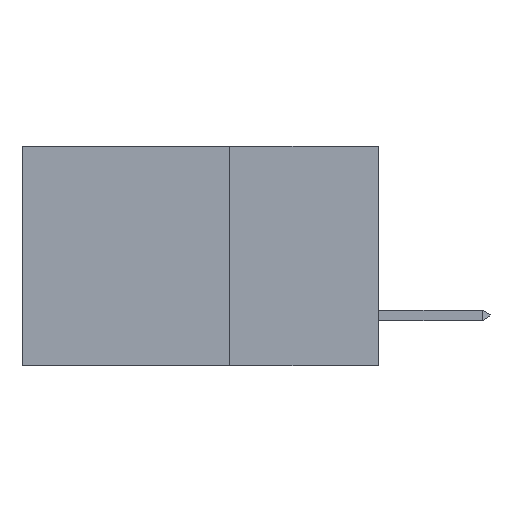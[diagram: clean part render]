
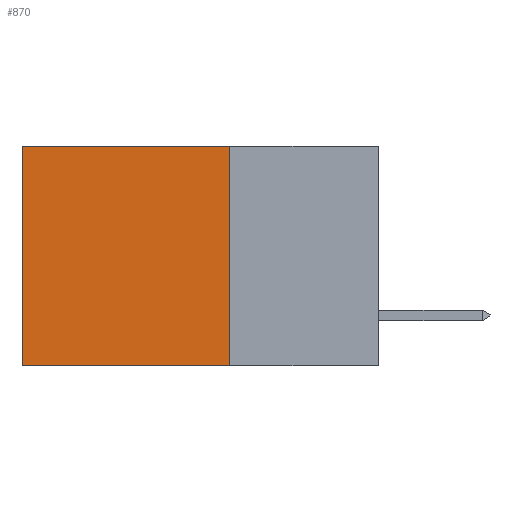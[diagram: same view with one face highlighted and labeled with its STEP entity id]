
A CAD part, left-side view. The second image highlights one B-rep face of the part: STEP entity #870.
In plain terms, the highlighted planar face has unit normal (-1, 0, 0).
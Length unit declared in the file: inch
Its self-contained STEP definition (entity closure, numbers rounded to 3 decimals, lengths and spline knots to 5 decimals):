
#489 = CARTESIAN_POINT ( 'NONE',  ( 0.2615, 0.25, -0.37 ) ) ;
#870 = ADVANCED_FACE ( 'NONE', ( #1251 ), #12846, .F. ) ;
#1251 = FACE_OUTER_BOUND ( 'NONE', #7239, .T. ) ;
#1718 = DIRECTION ( 'NONE',  ( 0., 0., -1. ) ) ;
#2157 = VERTEX_POINT ( 'NONE', #23594 ) ;
#2857 = DIRECTION ( 'NONE',  ( 0., 1., 0. ) ) ;
#4515 = VECTOR ( 'NONE', #1718, 39.37008 ) ;
#4715 = EDGE_CURVE ( 'NONE', #17413, #2157, #18904, .T. ) ;
#4854 = ORIENTED_EDGE ( 'NONE', *, *, #4715, .T. ) ;
#5540 = ORIENTED_EDGE ( 'NONE', *, *, #9986, .F. ) ;
#5983 = DIRECTION ( 'NONE',  ( 0., 1., 0. ) ) ;
#6253 = CARTESIAN_POINT ( 'NONE',  ( 0.2615, 0.25, 0. ) ) ;
#7239 = EDGE_LOOP ( 'NONE', ( #4854, #7318, #5540, #17774 ) ) ;
#7304 = CARTESIAN_POINT ( 'NONE',  ( 0.2615, 0.25, -0.37 ) ) ;
#7318 = ORIENTED_EDGE ( 'NONE', *, *, #13810, .F. ) ;
#7682 = EDGE_CURVE ( 'NONE', #24602, #17413, #10675, .T. ) ;
#8268 = VECTOR ( 'NONE', #18777, 39.37008 ) ;
#9056 = CARTESIAN_POINT ( 'NONE',  ( 0.2615, 0.25, -0.37 ) ) ;
#9926 = LINE ( 'NONE', #15931, #18428 ) ;
#9986 = EDGE_CURVE ( 'NONE', #24602, #16243, #13060, .T. ) ;
#10623 = AXIS2_PLACEMENT_3D ( 'NONE', #9056, #24739, #24611 ) ;
#10675 = LINE ( 'NONE', #22923, #18269 ) ;
#12846 = PLANE ( 'NONE',  #10623 ) ;
#13060 = LINE ( 'NONE', #7304, #4515 ) ;
#13810 = EDGE_CURVE ( 'NONE', #16243, #2157, #9926, .T. ) ;
#15931 = CARTESIAN_POINT ( 'NONE',  ( 0.2615, 0.25, -0.37 ) ) ;
#16243 = VERTEX_POINT ( 'NONE', #489 ) ;
#17069 = CARTESIAN_POINT ( 'NONE',  ( 0.2615, 0.6, -0.37 ) ) ;
#17413 = VERTEX_POINT ( 'NONE', #19092 ) ;
#17774 = ORIENTED_EDGE ( 'NONE', *, *, #7682, .T. ) ;
#18269 = VECTOR ( 'NONE', #2857, 39.37008 ) ;
#18428 = VECTOR ( 'NONE', #5983, 39.37008 ) ;
#18777 = DIRECTION ( 'NONE',  ( 0., 0., -1. ) ) ;
#18904 = LINE ( 'NONE', #17069, #8268 ) ;
#19092 = CARTESIAN_POINT ( 'NONE',  ( 0.2615, 0.6, 0. ) ) ;
#22923 = CARTESIAN_POINT ( 'NONE',  ( 0.2615, 0.25, 0. ) ) ;
#23594 = CARTESIAN_POINT ( 'NONE',  ( 0.2615, 0.6, -0.37 ) ) ;
#24602 = VERTEX_POINT ( 'NONE', #6253 ) ;
#24611 = DIRECTION ( 'NONE',  ( 0., 0., -1. ) ) ;
#24739 = DIRECTION ( 'NONE',  ( 1., 0., 0. ) ) ;
